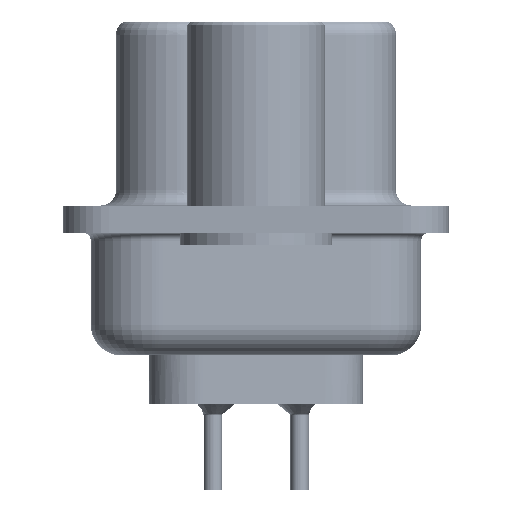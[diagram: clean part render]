
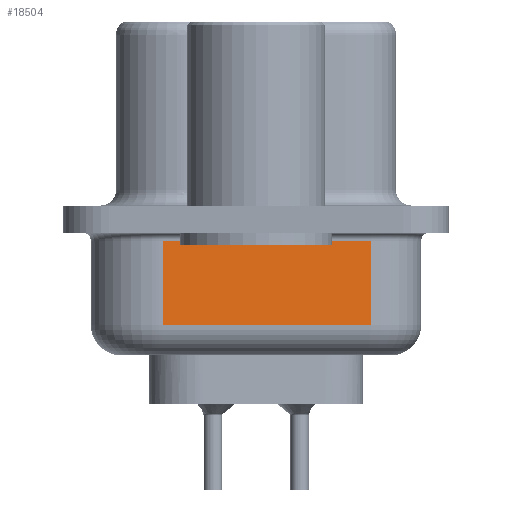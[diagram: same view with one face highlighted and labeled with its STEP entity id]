
A CAD part, left-side view. The second image highlights one B-rep face of the part: STEP entity #18504.
In plain terms, the highlighted planar face has unit normal (-0.985, -0.174, 0).
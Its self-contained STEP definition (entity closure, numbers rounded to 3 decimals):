
#1872 = DIRECTION ( 'NONE',  ( -0.174, 0.985, 0. ) ) ;
#3182 = AXIS2_PLACEMENT_3D ( 'NONE', #20421, #15928, #1872 ) ;
#3220 = DIRECTION ( 'NONE',  ( 0.174, -0.985, 0. ) ) ;
#3870 = VERTEX_POINT ( 'NONE', #30278 ) ;
#3893 = EDGE_LOOP ( 'NONE', ( #12392, #5917, #22218, #8408 ) ) ;
#4788 = EDGE_CURVE ( 'NONE', #26311, #13497, #12106, .T. ) ;
#5017 = EDGE_CURVE ( 'NONE', #26311, #20977, #6986, .T. ) ;
#5901 = VECTOR ( 'NONE', #29767, 1000. ) ;
#5917 = ORIENTED_EDGE ( 'NONE', *, *, #5017, .T. ) ;
#6986 = LINE ( 'NONE', #10838, #17848 ) ;
#7726 = CARTESIAN_POINT ( 'NONE',  ( 2.88, 3.053, -0.7 ) ) ;
#8408 = ORIENTED_EDGE ( 'NONE', *, *, #16498, .T. ) ;
#10838 = CARTESIAN_POINT ( 'NONE',  ( 2.88, 3.053, -3.45 ) ) ;
#12106 = LINE ( 'NONE', #29465, #5901 ) ;
#12392 = ORIENTED_EDGE ( 'NONE', *, *, #4788, .F. ) ;
#12662 = VECTOR ( 'NONE', #25244, 1000. ) ;
#13497 = VERTEX_POINT ( 'NONE', #22503 ) ;
#14732 = DIRECTION ( 'NONE',  ( -0.174, 0.985, 0. ) ) ;
#15928 = DIRECTION ( 'NONE',  ( 0.985, 0.174, 0. ) ) ;
#16498 = EDGE_CURVE ( 'NONE', #3870, #13497, #23049, .T. ) ;
#16981 = VECTOR ( 'NONE', #14732, 1000. ) ;
#17811 = FACE_OUTER_BOUND ( 'NONE', #3893, .T. ) ;
#17848 = VECTOR ( 'NONE', #3220, 1000. ) ;
#18504 = ADVANCED_FACE ( 'NONE', ( #17811 ), #27457, .F. ) ;
#19227 = CARTESIAN_POINT ( 'NONE',  ( 4.079, -3.747, -3.45 ) ) ;
#19449 = LINE ( 'NONE', #27687, #12662 ) ;
#20421 = CARTESIAN_POINT ( 'NONE',  ( 2.88, 3.053, -4.45 ) ) ;
#20749 = EDGE_CURVE ( 'NONE', #20977, #3870, #19449, .T. ) ;
#20977 = VERTEX_POINT ( 'NONE', #19227 ) ;
#22218 = ORIENTED_EDGE ( 'NONE', *, *, #20749, .T. ) ;
#22503 = CARTESIAN_POINT ( 'NONE',  ( 2.88, 3.053, -0.7 ) ) ;
#23049 = LINE ( 'NONE', #7726, #16981 ) ;
#25244 = DIRECTION ( 'NONE',  ( 0., 0., 1. ) ) ;
#26311 = VERTEX_POINT ( 'NONE', #28907 ) ;
#27457 = PLANE ( 'NONE',  #3182 ) ;
#27687 = CARTESIAN_POINT ( 'NONE',  ( 4.079, -3.747, -4.45 ) ) ;
#28907 = CARTESIAN_POINT ( 'NONE',  ( 2.88, 3.053, -3.45 ) ) ;
#29465 = CARTESIAN_POINT ( 'NONE',  ( 2.88, 3.053, -4.45 ) ) ;
#29767 = DIRECTION ( 'NONE',  ( 0., 0., 1. ) ) ;
#30278 = CARTESIAN_POINT ( 'NONE',  ( 4.079, -3.747, -0.7 ) ) ;
